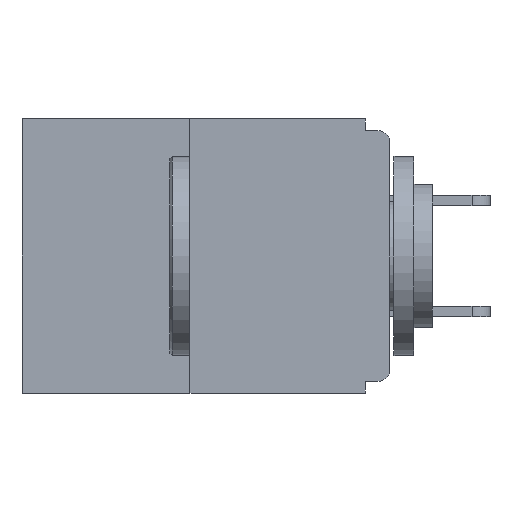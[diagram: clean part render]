
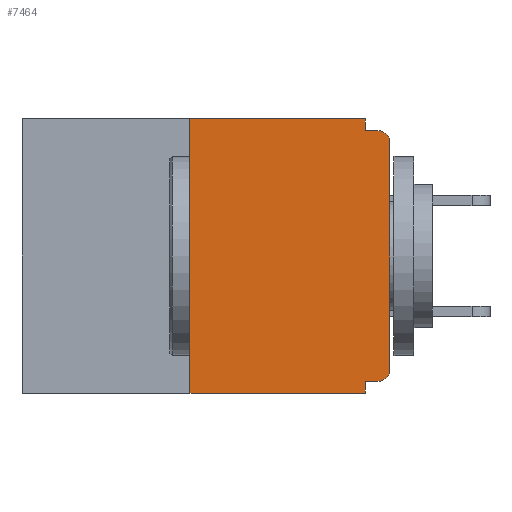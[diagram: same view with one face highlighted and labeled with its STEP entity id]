
A CAD part, left-side view. The second image highlights one B-rep face of the part: STEP entity #7464.
In plain terms, the highlighted planar face has unit normal (-1, 0, 0).
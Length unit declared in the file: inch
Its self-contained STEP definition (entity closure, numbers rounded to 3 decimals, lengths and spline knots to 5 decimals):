
#180 = DIRECTION ( 'NONE',  ( 0., -1., 0. ) ) ;
#496 = ORIENTED_EDGE ( 'NONE', *, *, #26220, .F. ) ;
#519 = CARTESIAN_POINT ( 'NONE',  ( 0., 0.25, 0. ) ) ;
#812 = VERTEX_POINT ( 'NONE', #10802 ) ;
#1175 = DIRECTION ( 'NONE',  ( 0., -1., 0. ) ) ;
#1213 = VERTEX_POINT ( 'NONE', #3486 ) ;
#1415 = PLANE ( 'NONE',  #12933 ) ;
#1481 = CARTESIAN_POINT ( 'NONE',  ( 0., 0.031, -0.328 ) ) ;
#1674 = LINE ( 'NONE', #13512, #22099 ) ;
#1778 = CARTESIAN_POINT ( 'NONE',  ( 0., 0., -0.03 ) ) ;
#2272 = VECTOR ( 'NONE', #5247, 39.37008 ) ;
#2635 = DIRECTION ( 'NONE',  ( 0., 0., -1. ) ) ;
#3314 = CARTESIAN_POINT ( 'NONE',  ( 0., 0., -0.313 ) ) ;
#3360 = ORIENTED_EDGE ( 'NONE', *, *, #21737, .F. ) ;
#3486 = CARTESIAN_POINT ( 'NONE',  ( 0., 0.25, -0.343 ) ) ;
#3655 = DIRECTION ( 'NONE',  ( -1., 0., 0. ) ) ;
#3682 = LINE ( 'NONE', #20101, #19216 ) ;
#4208 = VECTOR ( 'NONE', #26339, 39.37008 ) ;
#4426 = VERTEX_POINT ( 'NONE', #519 ) ;
#5195 = CIRCLE ( 'NONE', #27674, 0.015 ) ;
#5247 = DIRECTION ( 'NONE',  ( 0., -1., 0. ) ) ;
#5248 = VERTEX_POINT ( 'NONE', #15648 ) ;
#5803 = EDGE_CURVE ( 'NONE', #29115, #812, #22892, .T. ) ;
#5810 = VERTEX_POINT ( 'NONE', #25231 ) ;
#6957 = EDGE_CURVE ( 'NONE', #22979, #5810, #5195, .T. ) ;
#7464 = ADVANCED_FACE ( 'NONE', ( #14650 ), #1415, .F. ) ;
#8958 = EDGE_CURVE ( 'NONE', #5248, #11708, #15985, .T. ) ;
#9113 = VERTEX_POINT ( 'NONE', #1481 ) ;
#9717 = LINE ( 'NONE', #11724, #20326 ) ;
#10095 = CARTESIAN_POINT ( 'NONE',  ( 0., 0.46, 0. ) ) ;
#10385 = VECTOR ( 'NONE', #26609, 39.37008 ) ;
#10802 = CARTESIAN_POINT ( 'NONE',  ( 0., 0.031, -0.015 ) ) ;
#11708 = VERTEX_POINT ( 'NONE', #3314 ) ;
#11724 = CARTESIAN_POINT ( 'NONE',  ( 0., 0., 0. ) ) ;
#11763 = EDGE_CURVE ( 'NONE', #5248, #9113, #28806, .T. ) ;
#12376 = ORIENTED_EDGE ( 'NONE', *, *, #14491, .T. ) ;
#12933 = AXIS2_PLACEMENT_3D ( 'NONE', #15250, #19631, #17549 ) ;
#13281 = ORIENTED_EDGE ( 'NONE', *, *, #8958, .T. ) ;
#13512 = CARTESIAN_POINT ( 'NONE',  ( 0., 0.031, -0.343 ) ) ;
#13594 = VECTOR ( 'NONE', #1175, 39.37008 ) ;
#13804 = DIRECTION ( 'NONE',  ( 0., 0., -1. ) ) ;
#13860 = EDGE_CURVE ( 'NONE', #11708, #22979, #9717, .T. ) ;
#14317 = ORIENTED_EDGE ( 'NONE', *, *, #13860, .T. ) ;
#14491 = EDGE_CURVE ( 'NONE', #1213, #24231, #3682, .T. ) ;
#14650 = FACE_OUTER_BOUND ( 'NONE', #27835, .T. ) ;
#14823 = CARTESIAN_POINT ( 'NONE',  ( 0., 0.031, -0.343 ) ) ;
#15250 = CARTESIAN_POINT ( 'NONE',  ( 0., 0.46, 0. ) ) ;
#15648 = CARTESIAN_POINT ( 'NONE',  ( 0., 0.015, -0.328 ) ) ;
#15985 = CIRCLE ( 'NONE', #23355, 0.015 ) ;
#17020 = DIRECTION ( 'NONE',  ( 0., 1., 0. ) ) ;
#17549 = DIRECTION ( 'NONE',  ( 0., 0., -1. ) ) ;
#17973 = ORIENTED_EDGE ( 'NONE', *, *, #5803, .F. ) ;
#19216 = VECTOR ( 'NONE', #180, 39.37008 ) ;
#19288 = CARTESIAN_POINT ( 'NONE',  ( 0., 0., -0.328 ) ) ;
#19631 = DIRECTION ( 'NONE',  ( 1., 0., 0. ) ) ;
#19728 = CARTESIAN_POINT ( 'NONE',  ( 0., 0.015, -0.03 ) ) ;
#19826 = ORIENTED_EDGE ( 'NONE', *, *, #20428, .F. ) ;
#20101 = CARTESIAN_POINT ( 'NONE',  ( 0., 0.46, -0.343 ) ) ;
#20132 = CARTESIAN_POINT ( 'NONE',  ( 0., 0.031, 0. ) ) ;
#20326 = VECTOR ( 'NONE', #27604, 39.37008 ) ;
#20428 = EDGE_CURVE ( 'NONE', #4426, #29115, #21763, .T. ) ;
#20684 = EDGE_CURVE ( 'NONE', #9113, #24231, #1674, .T. ) ;
#21337 = LINE ( 'NONE', #22356, #10385 ) ;
#21737 = EDGE_CURVE ( 'NONE', #812, #5810, #25891, .T. ) ;
#21763 = LINE ( 'NONE', #10095, #13594 ) ;
#22099 = VECTOR ( 'NONE', #13804, 39.37008 ) ;
#22313 = ORIENTED_EDGE ( 'NONE', *, *, #20684, .F. ) ;
#22356 = CARTESIAN_POINT ( 'NONE',  ( 0., 0.25, 0. ) ) ;
#22892 = LINE ( 'NONE', #24941, #4208 ) ;
#22979 = VERTEX_POINT ( 'NONE', #1778 ) ;
#23283 = CARTESIAN_POINT ( 'NONE',  ( 0., 0., -0.015 ) ) ;
#23355 = AXIS2_PLACEMENT_3D ( 'NONE', #25413, #25111, #2635 ) ;
#23913 = VECTOR ( 'NONE', #17020, 39.37008 ) ;
#24231 = VERTEX_POINT ( 'NONE', #14823 ) ;
#24858 = ORIENTED_EDGE ( 'NONE', *, *, #6957, .T. ) ;
#24941 = CARTESIAN_POINT ( 'NONE',  ( 0., 0.031, 0. ) ) ;
#25111 = DIRECTION ( 'NONE',  ( -1., 0., 0. ) ) ;
#25231 = CARTESIAN_POINT ( 'NONE',  ( 0., 0.015, -0.015 ) ) ;
#25413 = CARTESIAN_POINT ( 'NONE',  ( 0., 0.015, -0.313 ) ) ;
#25851 = ORIENTED_EDGE ( 'NONE', *, *, #11763, .F. ) ;
#25891 = LINE ( 'NONE', #23283, #2272 ) ;
#26220 = EDGE_CURVE ( 'NONE', #1213, #4426, #21337, .T. ) ;
#26339 = DIRECTION ( 'NONE',  ( 0., 0., -1. ) ) ;
#26609 = DIRECTION ( 'NONE',  ( 0., 0., 1. ) ) ;
#27604 = DIRECTION ( 'NONE',  ( 0., 0., 1. ) ) ;
#27674 = AXIS2_PLACEMENT_3D ( 'NONE', #19728, #3655, #28572 ) ;
#27835 = EDGE_LOOP ( 'NONE', ( #19826, #496, #12376, #22313, #25851, #13281, #14317, #24858, #3360, #17973 ) ) ;
#28572 = DIRECTION ( 'NONE',  ( 0., 0., -1. ) ) ;
#28806 = LINE ( 'NONE', #19288, #23913 ) ;
#29115 = VERTEX_POINT ( 'NONE', #20132 ) ;
